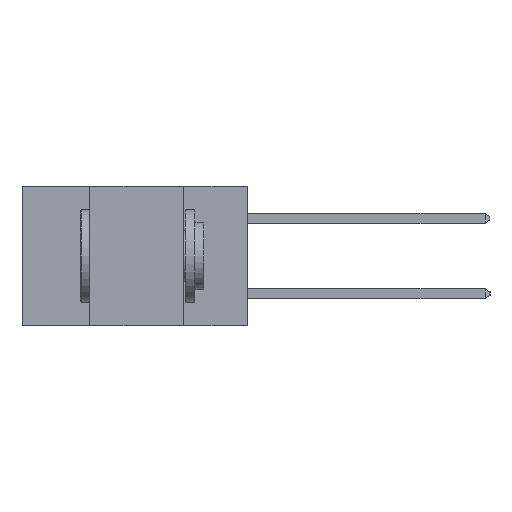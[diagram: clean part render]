
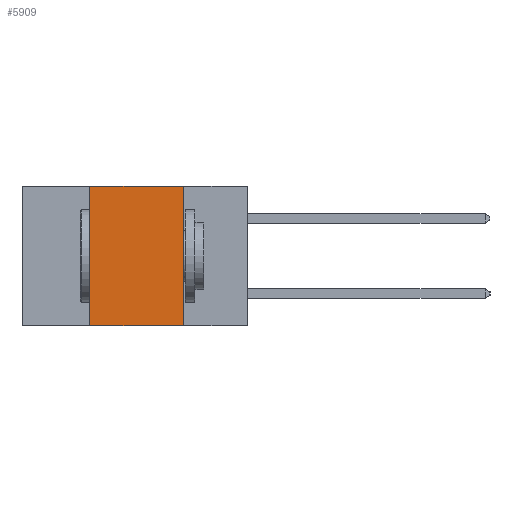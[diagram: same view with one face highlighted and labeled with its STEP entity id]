
A CAD part, left-side view. The second image highlights one B-rep face of the part: STEP entity #5909.
In plain terms, the highlighted planar face has unit normal (-1, 0, 0).
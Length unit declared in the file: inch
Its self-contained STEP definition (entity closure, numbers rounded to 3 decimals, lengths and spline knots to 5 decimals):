
#123 = CARTESIAN_POINT ( 'NONE',  ( 0., 0.17, 0. ) ) ;
#349 = CARTESIAN_POINT ( 'NONE',  ( 0., 0.6, 0. ) ) ;
#1639 = LINE ( 'NONE', #13585, #13396 ) ;
#1650 = LINE ( 'NONE', #2492, #7023 ) ;
#2099 = FACE_OUTER_BOUND ( 'NONE', #4151, .T. ) ;
#2117 = EDGE_CURVE ( 'NONE', #2917, #6475, #1650, .T. ) ;
#2492 = CARTESIAN_POINT ( 'NONE',  ( 0., 0.42, -0.37 ) ) ;
#2917 = VERTEX_POINT ( 'NONE', #5417 ) ;
#3883 = DIRECTION ( 'NONE',  ( 0., 0., 1. ) ) ;
#4151 = EDGE_LOOP ( 'NONE', ( #14761, #5590, #5988, #12421 ) ) ;
#4189 = EDGE_CURVE ( 'NONE', #6475, #12373, #15430, .T. ) ;
#4658 = DIRECTION ( 'NONE',  ( 0., 0., -1. ) ) ;
#4663 = VECTOR ( 'NONE', #8408, 39.37008 ) ;
#4758 = DIRECTION ( 'NONE',  ( 1., 0., 0. ) ) ;
#4782 = PLANE ( 'NONE',  #12466 ) ;
#4844 = CARTESIAN_POINT ( 'NONE',  ( 0., 0.6, 0. ) ) ;
#5417 = CARTESIAN_POINT ( 'NONE',  ( 0., 0.42, -0.37 ) ) ;
#5590 = ORIENTED_EDGE ( 'NONE', *, *, #4189, .F. ) ;
#5909 = ADVANCED_FACE ( 'NONE', ( #2099 ), #4782, .F. ) ;
#5988 = ORIENTED_EDGE ( 'NONE', *, *, #2117, .F. ) ;
#6004 = VECTOR ( 'NONE', #15083, 39.37008 ) ;
#6475 = VERTEX_POINT ( 'NONE', #9137 ) ;
#7023 = VECTOR ( 'NONE', #3883, 39.37008 ) ;
#7155 = LINE ( 'NONE', #8377, #4663 ) ;
#7339 = VERTEX_POINT ( 'NONE', #14284 ) ;
#8377 = CARTESIAN_POINT ( 'NONE',  ( 0., 0.6, -0.37 ) ) ;
#8408 = DIRECTION ( 'NONE',  ( 0., -1., 0. ) ) ;
#9076 = EDGE_CURVE ( 'NONE', #12373, #7339, #1639, .T. ) ;
#9137 = CARTESIAN_POINT ( 'NONE',  ( 0., 0.42, 0. ) ) ;
#11386 = EDGE_CURVE ( 'NONE', #2917, #7339, #7155, .T. ) ;
#12373 = VERTEX_POINT ( 'NONE', #123 ) ;
#12421 = ORIENTED_EDGE ( 'NONE', *, *, #11386, .T. ) ;
#12466 = AXIS2_PLACEMENT_3D ( 'NONE', #4844, #4758, #4658 ) ;
#13396 = VECTOR ( 'NONE', #14066, 39.37008 ) ;
#13585 = CARTESIAN_POINT ( 'NONE',  ( 0., 0.17, -0.37 ) ) ;
#14066 = DIRECTION ( 'NONE',  ( 0., 0., -1. ) ) ;
#14284 = CARTESIAN_POINT ( 'NONE',  ( 0., 0.17, -0.37 ) ) ;
#14761 = ORIENTED_EDGE ( 'NONE', *, *, #9076, .F. ) ;
#15083 = DIRECTION ( 'NONE',  ( 0., -1., 0. ) ) ;
#15430 = LINE ( 'NONE', #349, #6004 ) ;
